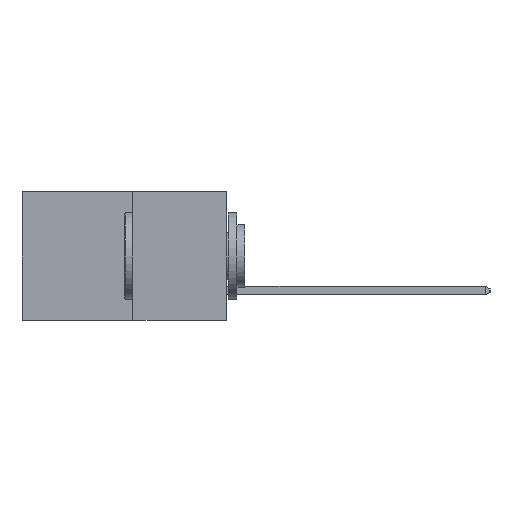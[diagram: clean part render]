
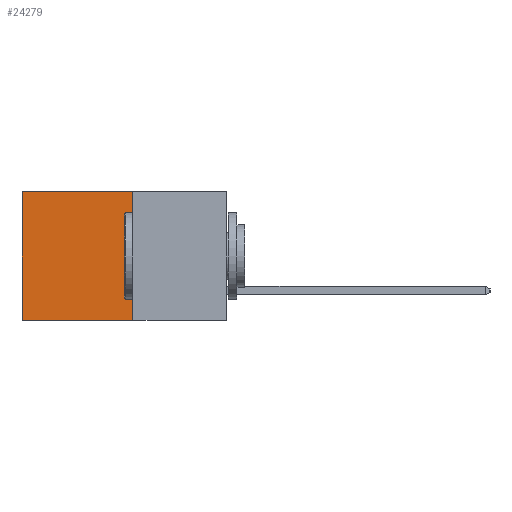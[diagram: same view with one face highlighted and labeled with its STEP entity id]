
A CAD part, left-side view. The second image highlights one B-rep face of the part: STEP entity #24279.
In plain terms, the highlighted planar face has unit normal (-1, 0, 0).
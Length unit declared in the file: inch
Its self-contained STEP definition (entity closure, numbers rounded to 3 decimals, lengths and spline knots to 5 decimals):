
#647 = VERTEX_POINT ( 'NONE', #18816 ) ;
#2526 = CARTESIAN_POINT ( 'NONE',  ( 0.277, 0.27, 0. ) ) ;
#3663 = CARTESIAN_POINT ( 'NONE',  ( 0.277, 0.27, -0.37 ) ) ;
#3766 = VECTOR ( 'NONE', #4758, 39.37008 ) ;
#4758 = DIRECTION ( 'NONE',  ( 0., 1., 0. ) ) ;
#5608 = VECTOR ( 'NONE', #10590, 39.37008 ) ;
#5922 = AXIS2_PLACEMENT_3D ( 'NONE', #17346, #19522, #6599 ) ;
#6599 = DIRECTION ( 'NONE',  ( 0., 0., -1. ) ) ;
#8390 = CARTESIAN_POINT ( 'NONE',  ( 0.277, 0.59, -0.37 ) ) ;
#8785 = ORIENTED_EDGE ( 'NONE', *, *, #18999, .F. ) ;
#9591 = CARTESIAN_POINT ( 'NONE',  ( 0.277, 0.27, -0.37 ) ) ;
#10235 = DIRECTION ( 'NONE',  ( 0., 0., -1. ) ) ;
#10579 = VECTOR ( 'NONE', #11758, 39.37008 ) ;
#10590 = DIRECTION ( 'NONE',  ( 0., 0., -1. ) ) ;
#11255 = LINE ( 'NONE', #9591, #10579 ) ;
#11710 = VECTOR ( 'NONE', #10235, 39.37008 ) ;
#11758 = DIRECTION ( 'NONE',  ( 0., 1., 0. ) ) ;
#12033 = LINE ( 'NONE', #8390, #5608 ) ;
#13728 = LINE ( 'NONE', #3663, #11710 ) ;
#14279 = CARTESIAN_POINT ( 'NONE',  ( 0.277, 0.27, -0.37 ) ) ;
#15159 = PLANE ( 'NONE',  #5922 ) ;
#15367 = CARTESIAN_POINT ( 'NONE',  ( 0.277, 0.59, 0. ) ) ;
#15929 = EDGE_CURVE ( 'NONE', #647, #23791, #21019, .T. ) ;
#16083 = EDGE_CURVE ( 'NONE', #18194, #18599, #11255, .T. ) ;
#16477 = FACE_OUTER_BOUND ( 'NONE', #26971, .T. ) ;
#17346 = CARTESIAN_POINT ( 'NONE',  ( 0.277, 0.27, -0.37 ) ) ;
#18194 = VERTEX_POINT ( 'NONE', #14279 ) ;
#18599 = VERTEX_POINT ( 'NONE', #21347 ) ;
#18816 = CARTESIAN_POINT ( 'NONE',  ( 0.277, 0.27, 0. ) ) ;
#18999 = EDGE_CURVE ( 'NONE', #647, #18194, #13728, .T. ) ;
#19522 = DIRECTION ( 'NONE',  ( 1., 0., 0. ) ) ;
#20938 = ORIENTED_EDGE ( 'NONE', *, *, #26259, .T. ) ;
#21019 = LINE ( 'NONE', #2526, #3766 ) ;
#21347 = CARTESIAN_POINT ( 'NONE',  ( 0.277, 0.59, -0.37 ) ) ;
#23791 = VERTEX_POINT ( 'NONE', #15367 ) ;
#24279 = ADVANCED_FACE ( 'NONE', ( #16477 ), #15159, .F. ) ;
#24644 = ORIENTED_EDGE ( 'NONE', *, *, #16083, .F. ) ;
#26259 = EDGE_CURVE ( 'NONE', #23791, #18599, #12033, .T. ) ;
#26390 = ORIENTED_EDGE ( 'NONE', *, *, #15929, .T. ) ;
#26971 = EDGE_LOOP ( 'NONE', ( #20938, #24644, #8785, #26390 ) ) ;
